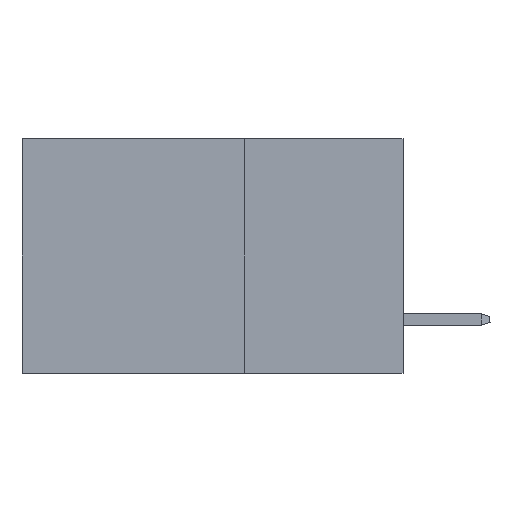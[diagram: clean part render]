
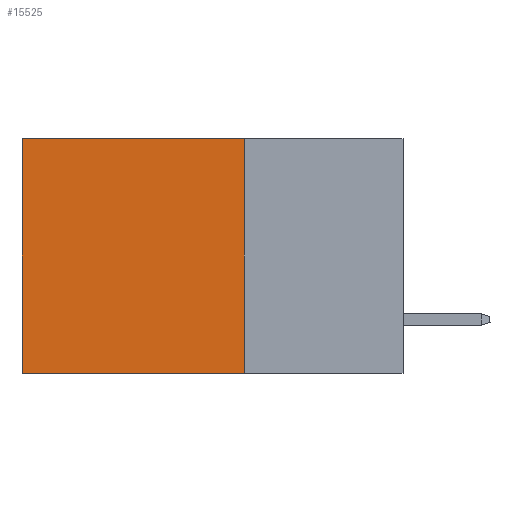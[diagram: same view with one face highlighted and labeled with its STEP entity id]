
A CAD part, left-side view. The second image highlights one B-rep face of the part: STEP entity #15525.
In plain terms, the highlighted planar face has unit normal (-1, 0, 0).
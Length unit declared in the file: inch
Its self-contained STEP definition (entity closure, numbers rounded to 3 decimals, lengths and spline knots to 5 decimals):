
#139 = DIRECTION ( 'NONE',  ( 0., 1., 0. ) ) ;
#233 = DIRECTION ( 'NONE',  ( 1., 0., 0. ) ) ;
#473 = CARTESIAN_POINT ( 'NONE',  ( 0.2875, 0.6, 0. ) ) ;
#1380 = DIRECTION ( 'NONE',  ( 0., 1., 0. ) ) ;
#1935 = ORIENTED_EDGE ( 'NONE', *, *, #11562, .F. ) ;
#1987 = EDGE_CURVE ( 'NONE', #26517, #13738, #13694, .T. ) ;
#2297 = CARTESIAN_POINT ( 'NONE',  ( 0.2875, 0.6, 0. ) ) ;
#2449 = CARTESIAN_POINT ( 'NONE',  ( 0.2875, 0.25, -0.37 ) ) ;
#2688 = ORIENTED_EDGE ( 'NONE', *, *, #25086, .F. ) ;
#4560 = CARTESIAN_POINT ( 'NONE',  ( 0.2875, 0.25, 0. ) ) ;
#6243 = LINE ( 'NONE', #2449, #25749 ) ;
#6275 = EDGE_CURVE ( 'NONE', #13738, #16757, #21442, .T. ) ;
#6722 = DIRECTION ( 'NONE',  ( 0., 0., -1. ) ) ;
#8492 = DIRECTION ( 'NONE',  ( 0., 0., -1. ) ) ;
#9316 = EDGE_LOOP ( 'NONE', ( #10193, #1935, #2688, #15361 ) ) ;
#10193 = ORIENTED_EDGE ( 'NONE', *, *, #6275, .T. ) ;
#10256 = VERTEX_POINT ( 'NONE', #12957 ) ;
#10515 = FACE_OUTER_BOUND ( 'NONE', #9316, .T. ) ;
#10628 = DIRECTION ( 'NONE',  ( 0., 0., -1. ) ) ;
#11562 = EDGE_CURVE ( 'NONE', #10256, #16757, #6243, .T. ) ;
#12236 = VECTOR ( 'NONE', #1380, 39.37008 ) ;
#12469 = CARTESIAN_POINT ( 'NONE',  ( 0.2875, 0.6, -0.37 ) ) ;
#12957 = CARTESIAN_POINT ( 'NONE',  ( 0.2875, 0.25, -0.37 ) ) ;
#13694 = LINE ( 'NONE', #19913, #12236 ) ;
#13738 = VERTEX_POINT ( 'NONE', #2297 ) ;
#15021 = AXIS2_PLACEMENT_3D ( 'NONE', #4560, #233, #8492 ) ;
#15361 = ORIENTED_EDGE ( 'NONE', *, *, #1987, .T. ) ;
#15525 = ADVANCED_FACE ( 'NONE', ( #10515 ), #18775, .F. ) ;
#16757 = VERTEX_POINT ( 'NONE', #12469 ) ;
#18775 = PLANE ( 'NONE',  #15021 ) ;
#19027 = CARTESIAN_POINT ( 'NONE',  ( 0.2875, 0.25, 0. ) ) ;
#19564 = LINE ( 'NONE', #19027, #21344 ) ;
#19913 = CARTESIAN_POINT ( 'NONE',  ( 0.2875, 0.25, 0. ) ) ;
#21344 = VECTOR ( 'NONE', #6722, 39.37008 ) ;
#21442 = LINE ( 'NONE', #473, #26299 ) ;
#25086 = EDGE_CURVE ( 'NONE', #26517, #10256, #19564, .T. ) ;
#25749 = VECTOR ( 'NONE', #139, 39.37008 ) ;
#26299 = VECTOR ( 'NONE', #10628, 39.37008 ) ;
#26351 = CARTESIAN_POINT ( 'NONE',  ( 0.2875, 0.25, 0. ) ) ;
#26517 = VERTEX_POINT ( 'NONE', #26351 ) ;
